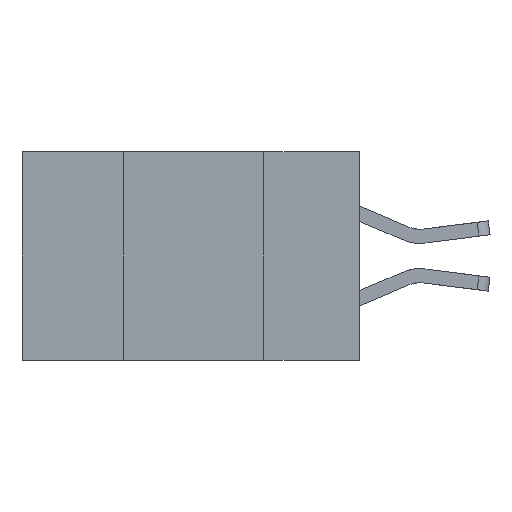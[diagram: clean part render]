
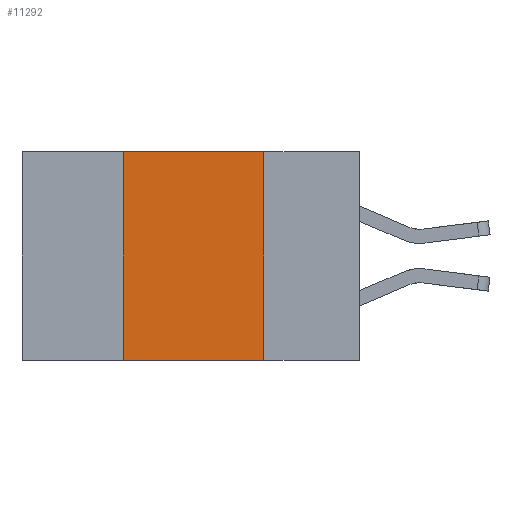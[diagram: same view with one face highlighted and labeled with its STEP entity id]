
A CAD part, left-side view. The second image highlights one B-rep face of the part: STEP entity #11292.
In plain terms, the highlighted planar face has unit normal (-1, 0, 0).
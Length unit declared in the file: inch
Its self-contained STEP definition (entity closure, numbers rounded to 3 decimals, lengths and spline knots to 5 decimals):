
#5 = VERTEX_POINT ( 'NONE', #12692 ) ;
#537 = DIRECTION ( 'NONE',  ( 0., -1., 0. ) ) ;
#606 = LINE ( 'NONE', #1747, #10512 ) ;
#954 = DIRECTION ( 'NONE',  ( 0., -1., 0. ) ) ;
#1061 = ORIENTED_EDGE ( 'NONE', *, *, #11235, .F. ) ;
#1217 = VERTEX_POINT ( 'NONE', #13472 ) ;
#1747 = CARTESIAN_POINT ( 'NONE',  ( 0., 0.42, 0. ) ) ;
#2049 = AXIS2_PLACEMENT_3D ( 'NONE', #7391, #2897, #9893 ) ;
#2501 = CARTESIAN_POINT ( 'NONE',  ( 0., 0.42, 0. ) ) ;
#2897 = DIRECTION ( 'NONE',  ( 1., 0., 0. ) ) ;
#3146 = EDGE_LOOP ( 'NONE', ( #10257, #1061, #14608, #7949 ) ) ;
#3822 = DIRECTION ( 'NONE',  ( 0., 0., -1. ) ) ;
#4603 = LINE ( 'NONE', #13866, #4732 ) ;
#4732 = VECTOR ( 'NONE', #3822, 39.37008 ) ;
#5471 = VECTOR ( 'NONE', #954, 39.37008 ) ;
#7391 = CARTESIAN_POINT ( 'NONE',  ( 0., 0.6, 0. ) ) ;
#7465 = CARTESIAN_POINT ( 'NONE',  ( 0., 0.6, 0. ) ) ;
#7681 = DIRECTION ( 'NONE',  ( 0., 0., 1. ) ) ;
#7949 = ORIENTED_EDGE ( 'NONE', *, *, #11819, .T. ) ;
#8398 = EDGE_CURVE ( 'NONE', #5, #11156, #606, .T. ) ;
#8533 = FACE_OUTER_BOUND ( 'NONE', #3146, .T. ) ;
#9113 = VECTOR ( 'NONE', #537, 39.37008 ) ;
#9249 = CARTESIAN_POINT ( 'NONE',  ( 0., 0.17, 0. ) ) ;
#9893 = DIRECTION ( 'NONE',  ( 0., 0., -1. ) ) ;
#10257 = ORIENTED_EDGE ( 'NONE', *, *, #12046, .F. ) ;
#10512 = VECTOR ( 'NONE', #7681, 39.37008 ) ;
#11156 = VERTEX_POINT ( 'NONE', #2501 ) ;
#11235 = EDGE_CURVE ( 'NONE', #11156, #14652, #11943, .T. ) ;
#11292 = ADVANCED_FACE ( 'NONE', ( #8533 ), #13304, .F. ) ;
#11819 = EDGE_CURVE ( 'NONE', #5, #1217, #12302, .T. ) ;
#11943 = LINE ( 'NONE', #7465, #9113 ) ;
#12046 = EDGE_CURVE ( 'NONE', #14652, #1217, #4603, .T. ) ;
#12302 = LINE ( 'NONE', #13422, #5471 ) ;
#12692 = CARTESIAN_POINT ( 'NONE',  ( 0., 0.42, -0.37 ) ) ;
#13304 = PLANE ( 'NONE',  #2049 ) ;
#13422 = CARTESIAN_POINT ( 'NONE',  ( 0., 0.6, -0.37 ) ) ;
#13472 = CARTESIAN_POINT ( 'NONE',  ( 0., 0.17, -0.37 ) ) ;
#13866 = CARTESIAN_POINT ( 'NONE',  ( 0., 0.17, 0. ) ) ;
#14608 = ORIENTED_EDGE ( 'NONE', *, *, #8398, .F. ) ;
#14652 = VERTEX_POINT ( 'NONE', #9249 ) ;
